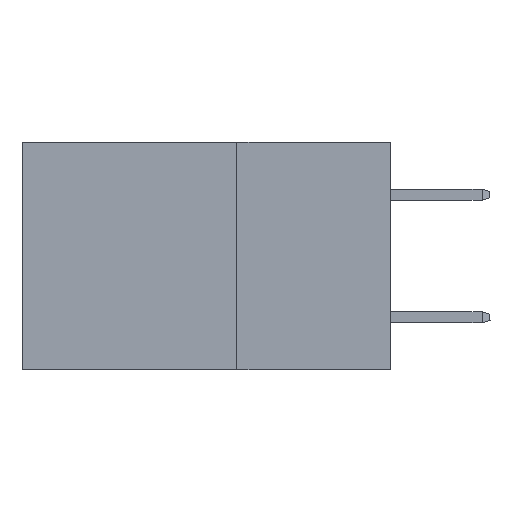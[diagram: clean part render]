
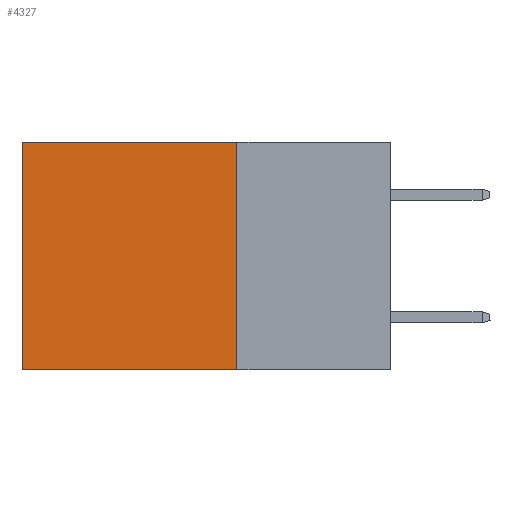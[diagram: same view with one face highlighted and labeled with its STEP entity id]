
A CAD part, left-side view. The second image highlights one B-rep face of the part: STEP entity #4327.
In plain terms, the highlighted planar face has unit normal (-1, 0, 0).
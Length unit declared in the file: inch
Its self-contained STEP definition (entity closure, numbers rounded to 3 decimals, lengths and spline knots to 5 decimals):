
#2963 = ORIENTED_EDGE ( 'NONE', *, *, #27319, .T. ) ;
#3400 = ORIENTED_EDGE ( 'NONE', *, *, #25481, .T. ) ;
#3885 = DIRECTION ( 'NONE',  ( 0., 0., -1. ) ) ;
#4321 = PLANE ( 'NONE',  #5944 ) ;
#4327 = ADVANCED_FACE ( 'NONE', ( #28895 ), #4321, .F. ) ;
#4534 = CARTESIAN_POINT ( 'NONE',  ( 0.2875, 0.25, -0.37 ) ) ;
#4734 = VERTEX_POINT ( 'NONE', #27915 ) ;
#4880 = LINE ( 'NONE', #14636, #23431 ) ;
#5944 = AXIS2_PLACEMENT_3D ( 'NONE', #7056, #12320, #16492 ) ;
#6052 = VECTOR ( 'NONE', #11221, 39.37008 ) ;
#6843 = VERTEX_POINT ( 'NONE', #18764 ) ;
#7056 = CARTESIAN_POINT ( 'NONE',  ( 0.2875, 0.25, 0. ) ) ;
#7349 = VECTOR ( 'NONE', #3885, 39.37008 ) ;
#7686 = DIRECTION ( 'NONE',  ( 0., 1., 0. ) ) ;
#9209 = CARTESIAN_POINT ( 'NONE',  ( 0.2875, 0.6, -0.37 ) ) ;
#9932 = LINE ( 'NONE', #29849, #11564 ) ;
#10953 = LINE ( 'NONE', #13789, #7349 ) ;
#11221 = DIRECTION ( 'NONE',  ( 0., 1., 0. ) ) ;
#11564 = VECTOR ( 'NONE', #7686, 39.37008 ) ;
#12320 = DIRECTION ( 'NONE',  ( 1., 0., 0. ) ) ;
#13789 = CARTESIAN_POINT ( 'NONE',  ( 0.2875, 0.25, 0. ) ) ;
#14636 = CARTESIAN_POINT ( 'NONE',  ( 0.2875, 0.6, 0. ) ) ;
#14775 = VERTEX_POINT ( 'NONE', #9209 ) ;
#16492 = DIRECTION ( 'NONE',  ( 0., 0., -1. ) ) ;
#17723 = EDGE_CURVE ( 'NONE', #6843, #25007, #10953, .T. ) ;
#17842 = ORIENTED_EDGE ( 'NONE', *, *, #31206, .F. ) ;
#18764 = CARTESIAN_POINT ( 'NONE',  ( 0.2875, 0.25, 0. ) ) ;
#19908 = EDGE_LOOP ( 'NONE', ( #3400, #17842, #22230, #2963 ) ) ;
#22230 = ORIENTED_EDGE ( 'NONE', *, *, #17723, .F. ) ;
#22694 = CARTESIAN_POINT ( 'NONE',  ( 0.2875, 0.25, -0.37 ) ) ;
#23431 = VECTOR ( 'NONE', #24362, 39.37008 ) ;
#24362 = DIRECTION ( 'NONE',  ( 0., 0., -1. ) ) ;
#25007 = VERTEX_POINT ( 'NONE', #4534 ) ;
#25481 = EDGE_CURVE ( 'NONE', #4734, #14775, #4880, .T. ) ;
#27319 = EDGE_CURVE ( 'NONE', #6843, #4734, #9932, .T. ) ;
#27915 = CARTESIAN_POINT ( 'NONE',  ( 0.2875, 0.6, 0. ) ) ;
#28096 = LINE ( 'NONE', #22694, #6052 ) ;
#28895 = FACE_OUTER_BOUND ( 'NONE', #19908, .T. ) ;
#29849 = CARTESIAN_POINT ( 'NONE',  ( 0.2875, 0.25, 0. ) ) ;
#31206 = EDGE_CURVE ( 'NONE', #25007, #14775, #28096, .T. ) ;
